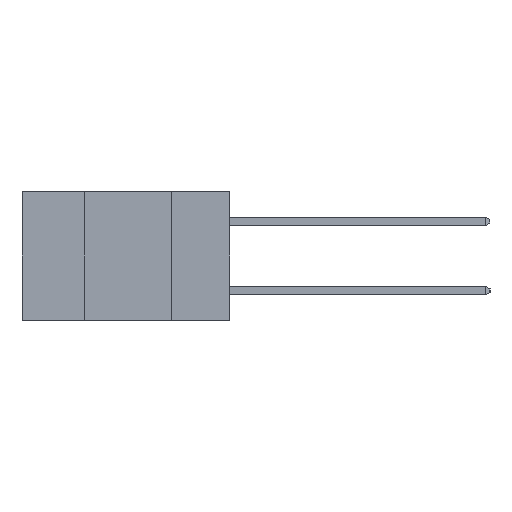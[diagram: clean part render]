
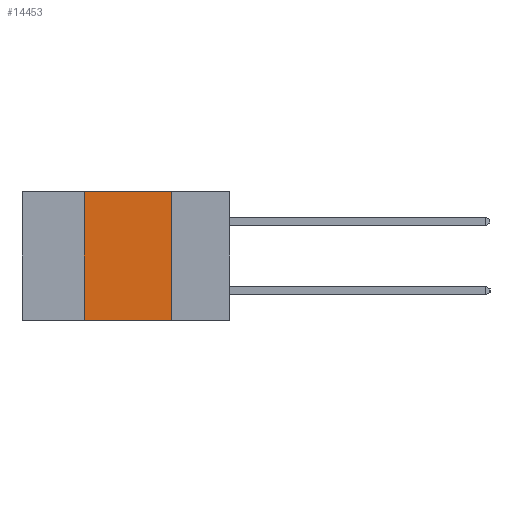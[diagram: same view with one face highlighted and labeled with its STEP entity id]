
A CAD part, left-side view. The second image highlights one B-rep face of the part: STEP entity #14453.
In plain terms, the highlighted planar face has unit normal (-1, 0, 0).
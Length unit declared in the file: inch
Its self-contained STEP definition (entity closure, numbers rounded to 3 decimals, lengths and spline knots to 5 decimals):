
#11 = CARTESIAN_POINT ( 'NONE',  ( 0., 0.6, -0.37 ) ) ;
#1151 = AXIS2_PLACEMENT_3D ( 'NONE', #9734, #4967, #15791 ) ;
#1506 = DIRECTION ( 'NONE',  ( 0., -1., 0. ) ) ;
#2543 = LINE ( 'NONE', #9544, #18483 ) ;
#2812 = EDGE_CURVE ( 'NONE', #5238, #19367, #15110, .T. ) ;
#3179 = DIRECTION ( 'NONE',  ( 0., -1., 0. ) ) ;
#3374 = PLANE ( 'NONE',  #1151 ) ;
#3397 = ORIENTED_EDGE ( 'NONE', *, *, #2812, .F. ) ;
#3536 = EDGE_CURVE ( 'NONE', #5238, #6755, #18330, .T. ) ;
#3905 = CARTESIAN_POINT ( 'NONE',  ( 0., 0.17, 0. ) ) ;
#4422 = VERTEX_POINT ( 'NONE', #3905 ) ;
#4850 = DIRECTION ( 'NONE',  ( 0., 0., 1. ) ) ;
#4967 = DIRECTION ( 'NONE',  ( 1., 0., 0. ) ) ;
#5238 = VERTEX_POINT ( 'NONE', #13002 ) ;
#6755 = VERTEX_POINT ( 'NONE', #11977 ) ;
#6854 = ORIENTED_EDGE ( 'NONE', *, *, #10835, .F. ) ;
#6910 = VECTOR ( 'NONE', #4850, 39.37008 ) ;
#7287 = FACE_OUTER_BOUND ( 'NONE', #9050, .T. ) ;
#9050 = EDGE_LOOP ( 'NONE', ( #6854, #15278, #3397, #17429 ) ) ;
#9544 = CARTESIAN_POINT ( 'NONE',  ( 0., 0.6, 0. ) ) ;
#9734 = CARTESIAN_POINT ( 'NONE',  ( 0., 0.6, 0. ) ) ;
#10033 = VECTOR ( 'NONE', #13085, 39.37008 ) ;
#10686 = CARTESIAN_POINT ( 'NONE',  ( 0., 0.42, -0.37 ) ) ;
#10835 = EDGE_CURVE ( 'NONE', #4422, #6755, #14084, .T. ) ;
#11977 = CARTESIAN_POINT ( 'NONE',  ( 0., 0.17, -0.37 ) ) ;
#13002 = CARTESIAN_POINT ( 'NONE',  ( 0., 0.42, -0.37 ) ) ;
#13085 = DIRECTION ( 'NONE',  ( 0., 0., -1. ) ) ;
#14064 = EDGE_CURVE ( 'NONE', #19367, #4422, #2543, .T. ) ;
#14084 = LINE ( 'NONE', #18979, #10033 ) ;
#14453 = ADVANCED_FACE ( 'NONE', ( #7287 ), #3374, .F. ) ;
#14840 = VECTOR ( 'NONE', #1506, 39.37008 ) ;
#15110 = LINE ( 'NONE', #10686, #6910 ) ;
#15278 = ORIENTED_EDGE ( 'NONE', *, *, #14064, .F. ) ;
#15791 = DIRECTION ( 'NONE',  ( 0., 0., -1. ) ) ;
#17429 = ORIENTED_EDGE ( 'NONE', *, *, #3536, .T. ) ;
#18330 = LINE ( 'NONE', #11, #14840 ) ;
#18483 = VECTOR ( 'NONE', #3179, 39.37008 ) ;
#18979 = CARTESIAN_POINT ( 'NONE',  ( 0., 0.17, -0.37 ) ) ;
#19367 = VERTEX_POINT ( 'NONE', #19911 ) ;
#19911 = CARTESIAN_POINT ( 'NONE',  ( 0., 0.42, 0. ) ) ;
